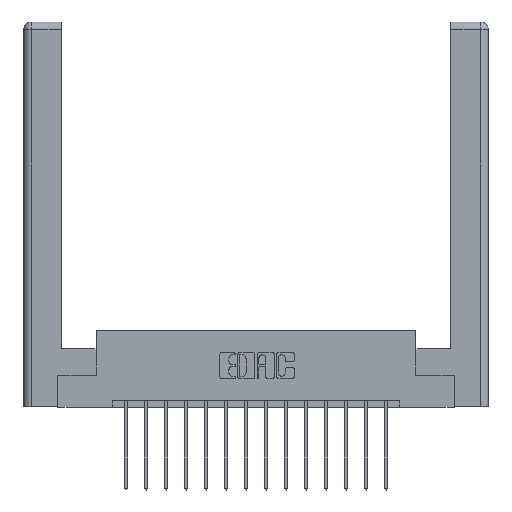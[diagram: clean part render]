
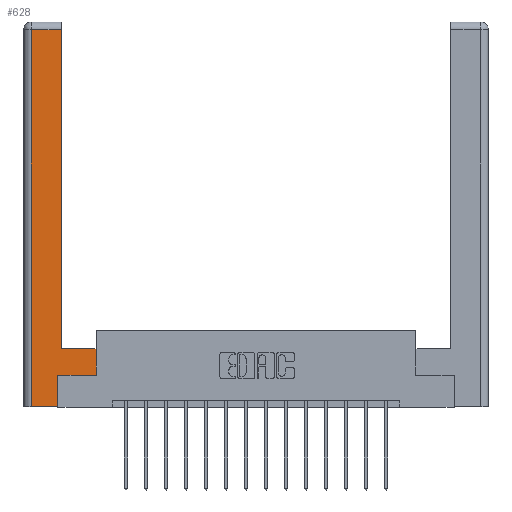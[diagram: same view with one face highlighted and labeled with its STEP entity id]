
A CAD part, top view. The second image highlights one B-rep face of the part: STEP entity #628.
In plain terms, the highlighted planar face has unit normal (0, 0, 1).
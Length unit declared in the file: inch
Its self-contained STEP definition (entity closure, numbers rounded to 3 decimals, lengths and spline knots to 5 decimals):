
#238 = CARTESIAN_POINT ( 'NONE',  ( 0.565, 0.45, 0. ) ) ;
#239 = DIRECTION ( 'NONE',  ( 1., 0., 0. ) ) ;
#438 = VERTEX_POINT ( 'NONE', #1781 ) ;
#628 = ADVANCED_FACE ( 'NONE', ( #16883 ), #9952, .F. ) ;
#744 = VECTOR ( 'NONE', #1261, 39.37008 ) ;
#1146 = DIRECTION ( 'NONE',  ( 0., 1., 0. ) ) ;
#1261 = DIRECTION ( 'NONE',  ( 0., -1., 0. ) ) ;
#1456 = CARTESIAN_POINT ( 'NONE',  ( 0.565, 0.45, 0. ) ) ;
#1666 = CARTESIAN_POINT ( 'NONE',  ( 0.265, 0., 0. ) ) ;
#1781 = CARTESIAN_POINT ( 'NONE',  ( 0.0615, 0., 0. ) ) ;
#1827 = CARTESIAN_POINT ( 'NONE',  ( 0.265, 0., 0. ) ) ;
#2083 = DIRECTION ( 'NONE',  ( 0., 0., -1. ) ) ;
#2445 = ORIENTED_EDGE ( 'NONE', *, *, #3291, .T. ) ;
#2560 = EDGE_CURVE ( 'NONE', #9659, #4205, #5625, .T. ) ;
#2813 = EDGE_CURVE ( 'NONE', #6182, #15283, #11784, .T. ) ;
#2942 = VECTOR ( 'NONE', #10200, 39.37008 ) ;
#3291 = EDGE_CURVE ( 'NONE', #438, #6182, #6020, .T. ) ;
#3348 = VECTOR ( 'NONE', #14354, 39.37008 ) ;
#3627 = VERTEX_POINT ( 'NONE', #238 ) ;
#3678 = ORIENTED_EDGE ( 'NONE', *, *, #2560, .T. ) ;
#3827 = LINE ( 'NONE', #12035, #9209 ) ;
#4205 = VERTEX_POINT ( 'NONE', #15961 ) ;
#4368 = DIRECTION ( 'NONE',  ( 1., 0., 0. ) ) ;
#5123 = CARTESIAN_POINT ( 'NONE',  ( 0.295, 0.45, 0. ) ) ;
#5201 = ORIENTED_EDGE ( 'NONE', *, *, #16458, .T. ) ;
#5323 = CARTESIAN_POINT ( 'NONE',  ( 0.0615, 0., 0. ) ) ;
#5436 = AXIS2_PLACEMENT_3D ( 'NONE', #7408, #2083, #11449 ) ;
#5526 = VECTOR ( 'NONE', #1146, 39.37008 ) ;
#5601 = CARTESIAN_POINT ( 'NONE',  ( 0.295, 2.94, 0. ) ) ;
#5625 = LINE ( 'NONE', #9141, #3348 ) ;
#5881 = EDGE_CURVE ( 'NONE', #4205, #438, #11490, .T. ) ;
#6020 = LINE ( 'NONE', #1666, #9128 ) ;
#6182 = VERTEX_POINT ( 'NONE', #1827 ) ;
#6429 = ORIENTED_EDGE ( 'NONE', *, *, #8792, .T. ) ;
#6653 = VECTOR ( 'NONE', #13875, 39.37008 ) ;
#7087 = LINE ( 'NONE', #1456, #6653 ) ;
#7408 = CARTESIAN_POINT ( 'NONE',  ( 0., 0., 0. ) ) ;
#7677 = DIRECTION ( 'NONE',  ( 0., 1., 0. ) ) ;
#8159 = LINE ( 'NONE', #5123, #2942 ) ;
#8792 = EDGE_CURVE ( 'NONE', #15283, #14179, #3827, .T. ) ;
#9128 = VECTOR ( 'NONE', #4368, 39.37008 ) ;
#9141 = CARTESIAN_POINT ( 'NONE',  ( 0.0615, 2.94, 0. ) ) ;
#9209 = VECTOR ( 'NONE', #239, 39.37008 ) ;
#9659 = VERTEX_POINT ( 'NONE', #5601 ) ;
#9952 = PLANE ( 'NONE',  #5436 ) ;
#10200 = DIRECTION ( 'NONE',  ( -1., 0., 0. ) ) ;
#10226 = CARTESIAN_POINT ( 'NONE',  ( 0.295, 0.45, 0. ) ) ;
#10275 = ORIENTED_EDGE ( 'NONE', *, *, #2813, .T. ) ;
#11449 = DIRECTION ( 'NONE',  ( -1., 0., 0. ) ) ;
#11490 = LINE ( 'NONE', #5323, #744 ) ;
#11573 = CARTESIAN_POINT ( 'NONE',  ( 0.265, 0.245, 0. ) ) ;
#11784 = LINE ( 'NONE', #15506, #16165 ) ;
#12035 = CARTESIAN_POINT ( 'NONE',  ( 0.565, 0.245, 0. ) ) ;
#13277 = EDGE_CURVE ( 'NONE', #3627, #14603, #8159, .T. ) ;
#13804 = LINE ( 'NONE', #17038, #5526 ) ;
#13815 = ORIENTED_EDGE ( 'NONE', *, *, #5881, .T. ) ;
#13875 = DIRECTION ( 'NONE',  ( 0., 1., 0. ) ) ;
#14179 = VERTEX_POINT ( 'NONE', #15865 ) ;
#14224 = EDGE_CURVE ( 'NONE', #14179, #3627, #7087, .T. ) ;
#14354 = DIRECTION ( 'NONE',  ( -1., 0., 0. ) ) ;
#14370 = ORIENTED_EDGE ( 'NONE', *, *, #13277, .T. ) ;
#14448 = EDGE_LOOP ( 'NONE', ( #5201, #3678, #13815, #2445, #10275, #6429, #16728, #14370 ) ) ;
#14603 = VERTEX_POINT ( 'NONE', #10226 ) ;
#15283 = VERTEX_POINT ( 'NONE', #11573 ) ;
#15506 = CARTESIAN_POINT ( 'NONE',  ( 0.265, 0.245, 0. ) ) ;
#15865 = CARTESIAN_POINT ( 'NONE',  ( 0.565, 0.245, 0. ) ) ;
#15961 = CARTESIAN_POINT ( 'NONE',  ( 0.0615, 2.94, 0. ) ) ;
#16165 = VECTOR ( 'NONE', #7677, 39.37008 ) ;
#16458 = EDGE_CURVE ( 'NONE', #14603, #9659, #13804, .T. ) ;
#16728 = ORIENTED_EDGE ( 'NONE', *, *, #14224, .T. ) ;
#16883 = FACE_OUTER_BOUND ( 'NONE', #14448, .T. ) ;
#17038 = CARTESIAN_POINT ( 'NONE',  ( 0.295, 3., 0. ) ) ;
